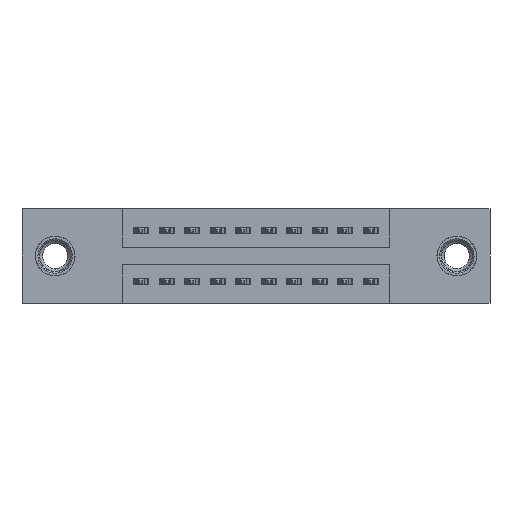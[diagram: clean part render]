
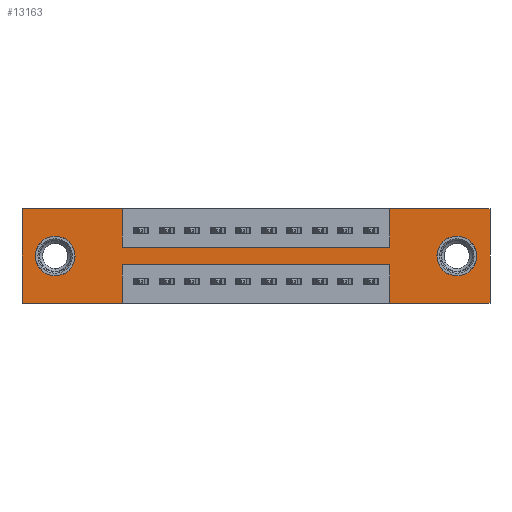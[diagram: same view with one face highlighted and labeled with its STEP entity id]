
A CAD part, front view. The second image highlights one B-rep face of the part: STEP entity #13163.
In plain terms, the highlighted planar face has unit normal (0, -1, 0).
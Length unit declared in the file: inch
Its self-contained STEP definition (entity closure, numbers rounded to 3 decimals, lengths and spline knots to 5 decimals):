
#22 = EDGE_CURVE ( 'NONE', #8082, #11016, #11154, .T. ) ;
#330 = CARTESIAN_POINT ( 'NONE',  ( 0.13, 0., -0.107 ) ) ;
#341 = LINE ( 'NONE', #5805, #5566 ) ;
#348 = CARTESIAN_POINT ( 'NONE',  ( 1.4425, 0., -0.15 ) ) ;
#742 = VERTEX_POINT ( 'NONE', #7881 ) ;
#766 = DIRECTION ( 'NONE',  ( 1., 0., 0. ) ) ;
#913 = EDGE_CURVE ( 'NONE', #10144, #1831, #9846, .T. ) ;
#1039 = EDGE_CURVE ( 'NONE', #12846, #10144, #13031, .T. ) ;
#1486 = CIRCLE ( 'NONE', #9671, 0.078 ) ;
#1671 = LINE ( 'NONE', #9073, #3831 ) ;
#1738 = VECTOR ( 'NONE', #3361, 39.37008 ) ;
#1769 = AXIS2_PLACEMENT_3D ( 'NONE', #9047, #1805, #11122 ) ;
#1805 = DIRECTION ( 'NONE',  ( 0., 1., 0. ) ) ;
#1831 = VERTEX_POINT ( 'NONE', #10173 ) ;
#1923 = CARTESIAN_POINT ( 'NONE',  ( 0.3925, 0., -0.22 ) ) ;
#1927 = LINE ( 'NONE', #7587, #1738 ) ;
#1950 = DIRECTION ( 'NONE',  ( -1., 0., 0. ) ) ;
#2017 = VECTOR ( 'NONE', #8834, 39.37008 ) ;
#2061 = ORIENTED_EDGE ( 'NONE', *, *, #11308, .F. ) ;
#2134 = CARTESIAN_POINT ( 'NONE',  ( 1.705, 0., -0.263 ) ) ;
#2552 = ORIENTED_EDGE ( 'NONE', *, *, #3732, .F. ) ;
#2582 = CARTESIAN_POINT ( 'NONE',  ( 0., 0., 0. ) ) ;
#2621 = VECTOR ( 'NONE', #9865, 39.37008 ) ;
#2636 = VECTOR ( 'NONE', #1950, 39.37008 ) ;
#2796 = ORIENTED_EDGE ( 'NONE', *, *, #13103, .F. ) ;
#3004 = CIRCLE ( 'NONE', #1769, 0.078 ) ;
#3109 = LINE ( 'NONE', #8820, #9702 ) ;
#3118 = EDGE_CURVE ( 'NONE', #12015, #9289, #3109, .T. ) ;
#3210 = CARTESIAN_POINT ( 'NONE',  ( 0., 0., -0.37 ) ) ;
#3249 = CARTESIAN_POINT ( 'NONE',  ( 0.13, 0., -0.185 ) ) ;
#3361 = DIRECTION ( 'NONE',  ( -1., 0., 0. ) ) ;
#3437 = CARTESIAN_POINT ( 'NONE',  ( 1.835, 0., -0.37 ) ) ;
#3732 = EDGE_CURVE ( 'NONE', #7843, #11007, #1927, .T. ) ;
#3734 = VECTOR ( 'NONE', #13028, 39.37008 ) ;
#3824 = LINE ( 'NONE', #4738, #2017 ) ;
#3831 = VECTOR ( 'NONE', #4975, 39.37008 ) ;
#3941 = CARTESIAN_POINT ( 'NONE',  ( 0.3925, 0., -0.15 ) ) ;
#4263 = FACE_BOUND ( 'NONE', #4465, .T. ) ;
#4465 = EDGE_LOOP ( 'NONE', ( #6788, #13098 ) ) ;
#4634 = AXIS2_PLACEMENT_3D ( 'NONE', #9168, #6195, #5168 ) ;
#4644 = EDGE_CURVE ( 'NONE', #11007, #6628, #12559, .T. ) ;
#4738 = CARTESIAN_POINT ( 'NONE',  ( 0.3925, 0., 0. ) ) ;
#4890 = LINE ( 'NONE', #12985, #2621 ) ;
#4975 = DIRECTION ( 'NONE',  ( 0., 0., -1. ) ) ;
#5049 = FACE_BOUND ( 'NONE', #7196, .T. ) ;
#5168 = DIRECTION ( 'NONE',  ( 0., 0., -1. ) ) ;
#5306 = EDGE_CURVE ( 'NONE', #9591, #5354, #5488, .T. ) ;
#5354 = VERTEX_POINT ( 'NONE', #330 ) ;
#5441 = ORIENTED_EDGE ( 'NONE', *, *, #22, .T. ) ;
#5488 = CIRCLE ( 'NONE', #12008, 0.078 ) ;
#5550 = ORIENTED_EDGE ( 'NONE', *, *, #3118, .F. ) ;
#5566 = VECTOR ( 'NONE', #766, 39.37008 ) ;
#5805 = CARTESIAN_POINT ( 'NONE',  ( 0., 0., 0. ) ) ;
#6195 = DIRECTION ( 'NONE',  ( 0., 1., 0. ) ) ;
#6290 = CARTESIAN_POINT ( 'NONE',  ( 0.3925, 0., -0.37 ) ) ;
#6348 = CARTESIAN_POINT ( 'NONE',  ( 1.4425, 0., 0. ) ) ;
#6370 = EDGE_LOOP ( 'NONE', ( #2796, #7929, #13135, #12585, #2061, #12685, #9750, #5550, #8366, #11106, #10973, #2552 ) ) ;
#6628 = VERTEX_POINT ( 'NONE', #9191 ) ;
#6699 = LINE ( 'NONE', #7328, #9110 ) ;
#6788 = ORIENTED_EDGE ( 'NONE', *, *, #12154, .T. ) ;
#6825 = CARTESIAN_POINT ( 'NONE',  ( 0., 0., -0.37 ) ) ;
#6924 = VECTOR ( 'NONE', #10322, 39.37008 ) ;
#6965 = CARTESIAN_POINT ( 'NONE',  ( 1.4425, 0., -0.37 ) ) ;
#7107 = VECTOR ( 'NONE', #12652, 39.37008 ) ;
#7196 = EDGE_LOOP ( 'NONE', ( #7478, #5441 ) ) ;
#7272 = DIRECTION ( 'NONE',  ( 0., 0., 1. ) ) ;
#7328 = CARTESIAN_POINT ( 'NONE',  ( 1.4425, 0., 0. ) ) ;
#7478 = ORIENTED_EDGE ( 'NONE', *, *, #11907, .T. ) ;
#7511 = AXIS2_PLACEMENT_3D ( 'NONE', #6825, #10111, #10024 ) ;
#7587 = CARTESIAN_POINT ( 'NONE',  ( 0., 0., -0.37 ) ) ;
#7719 = EDGE_CURVE ( 'NONE', #11239, #12967, #341, .T. ) ;
#7843 = VERTEX_POINT ( 'NONE', #6290 ) ;
#7881 = CARTESIAN_POINT ( 'NONE',  ( 0.3925, 0., 0. ) ) ;
#7929 = ORIENTED_EDGE ( 'NONE', *, *, #8216, .F. ) ;
#8082 = VERTEX_POINT ( 'NONE', #2134 ) ;
#8216 = EDGE_CURVE ( 'NONE', #1831, #10260, #12606, .T. ) ;
#8305 = DIRECTION ( 'NONE',  ( 0., 0., 1. ) ) ;
#8366 = ORIENTED_EDGE ( 'NONE', *, *, #11687, .F. ) ;
#8448 = CARTESIAN_POINT ( 'NONE',  ( 0.13, 0., -0.185 ) ) ;
#8820 = CARTESIAN_POINT ( 'NONE',  ( 0.3925, 0., -0.15 ) ) ;
#8834 = DIRECTION ( 'NONE',  ( 0., 0., -1. ) ) ;
#9047 = CARTESIAN_POINT ( 'NONE',  ( 1.705, 0., -0.185 ) ) ;
#9073 = CARTESIAN_POINT ( 'NONE',  ( 1.835, 0., 0. ) ) ;
#9084 = CARTESIAN_POINT ( 'NONE',  ( 0.13, 0., -0.263 ) ) ;
#9110 = VECTOR ( 'NONE', #8305, 39.37008 ) ;
#9146 = EDGE_CURVE ( 'NONE', #6628, #742, #12037, .T. ) ;
#9168 = CARTESIAN_POINT ( 'NONE',  ( 1.705, 0., -0.185 ) ) ;
#9191 = CARTESIAN_POINT ( 'NONE',  ( 0., 0., 0. ) ) ;
#9289 = VERTEX_POINT ( 'NONE', #348 ) ;
#9591 = VERTEX_POINT ( 'NONE', #9084 ) ;
#9671 = AXIS2_PLACEMENT_3D ( 'NONE', #8448, #10448, #12452 ) ;
#9702 = VECTOR ( 'NONE', #12943, 39.37008 ) ;
#9710 = CARTESIAN_POINT ( 'NONE',  ( 0., 0., -0.37 ) ) ;
#9750 = ORIENTED_EDGE ( 'NONE', *, *, #12176, .F. ) ;
#9846 = LINE ( 'NONE', #6965, #3734 ) ;
#9865 = DIRECTION ( 'NONE',  ( 0., 0., -1. ) ) ;
#10024 = DIRECTION ( 'NONE',  ( 0., 0., -1. ) ) ;
#10111 = DIRECTION ( 'NONE',  ( 0., -1., 0. ) ) ;
#10144 = VERTEX_POINT ( 'NONE', #11956 ) ;
#10173 = CARTESIAN_POINT ( 'NONE',  ( 1.4425, 0., -0.22 ) ) ;
#10260 = VERTEX_POINT ( 'NONE', #10589 ) ;
#10322 = DIRECTION ( 'NONE',  ( -1., 0., 0. ) ) ;
#10353 = DIRECTION ( 'NONE',  ( 0., 1., 0. ) ) ;
#10402 = CARTESIAN_POINT ( 'NONE',  ( 1.705, 0., -0.107 ) ) ;
#10448 = DIRECTION ( 'NONE',  ( 0., 1., 0. ) ) ;
#10589 = CARTESIAN_POINT ( 'NONE',  ( 0.3925, 0., -0.22 ) ) ;
#10627 = CARTESIAN_POINT ( 'NONE',  ( 1.835, 0., 0. ) ) ;
#10960 = VECTOR ( 'NONE', #11546, 39.37008 ) ;
#10973 = ORIENTED_EDGE ( 'NONE', *, *, #4644, .F. ) ;
#11007 = VERTEX_POINT ( 'NONE', #3210 ) ;
#11016 = VERTEX_POINT ( 'NONE', #10402 ) ;
#11106 = ORIENTED_EDGE ( 'NONE', *, *, #9146, .F. ) ;
#11122 = DIRECTION ( 'NONE',  ( 0., 0., -1. ) ) ;
#11154 = CIRCLE ( 'NONE', #4634, 0.078 ) ;
#11168 = FACE_OUTER_BOUND ( 'NONE', #6370, .T. ) ;
#11239 = VERTEX_POINT ( 'NONE', #6348 ) ;
#11308 = EDGE_CURVE ( 'NONE', #12967, #12846, #1671, .T. ) ;
#11546 = DIRECTION ( 'NONE',  ( 1., 0., 0. ) ) ;
#11687 = EDGE_CURVE ( 'NONE', #742, #12015, #3824, .T. ) ;
#11902 = PLANE ( 'NONE',  #7511 ) ;
#11907 = EDGE_CURVE ( 'NONE', #11016, #8082, #3004, .T. ) ;
#11956 = CARTESIAN_POINT ( 'NONE',  ( 1.4425, 0., -0.37 ) ) ;
#12008 = AXIS2_PLACEMENT_3D ( 'NONE', #3249, #10353, #7272 ) ;
#12015 = VERTEX_POINT ( 'NONE', #3941 ) ;
#12037 = LINE ( 'NONE', #12630, #10960 ) ;
#12154 = EDGE_CURVE ( 'NONE', #5354, #9591, #1486, .T. ) ;
#12176 = EDGE_CURVE ( 'NONE', #9289, #11239, #6699, .T. ) ;
#12452 = DIRECTION ( 'NONE',  ( 0., 0., 1. ) ) ;
#12559 = LINE ( 'NONE', #2582, #7107 ) ;
#12585 = ORIENTED_EDGE ( 'NONE', *, *, #1039, .F. ) ;
#12606 = LINE ( 'NONE', #1923, #2636 ) ;
#12630 = CARTESIAN_POINT ( 'NONE',  ( 0., 0., 0. ) ) ;
#12652 = DIRECTION ( 'NONE',  ( 0., 0., 1. ) ) ;
#12685 = ORIENTED_EDGE ( 'NONE', *, *, #7719, .F. ) ;
#12846 = VERTEX_POINT ( 'NONE', #3437 ) ;
#12943 = DIRECTION ( 'NONE',  ( 1., 0., 0. ) ) ;
#12967 = VERTEX_POINT ( 'NONE', #10627 ) ;
#12985 = CARTESIAN_POINT ( 'NONE',  ( 0.3925, 0., -0.37 ) ) ;
#13028 = DIRECTION ( 'NONE',  ( 0., 0., 1. ) ) ;
#13031 = LINE ( 'NONE', #9710, #6924 ) ;
#13098 = ORIENTED_EDGE ( 'NONE', *, *, #5306, .T. ) ;
#13103 = EDGE_CURVE ( 'NONE', #10260, #7843, #4890, .T. ) ;
#13135 = ORIENTED_EDGE ( 'NONE', *, *, #913, .F. ) ;
#13163 = ADVANCED_FACE ( 'NONE', ( #5049, #4263, #11168 ), #11902, .T. ) ;
